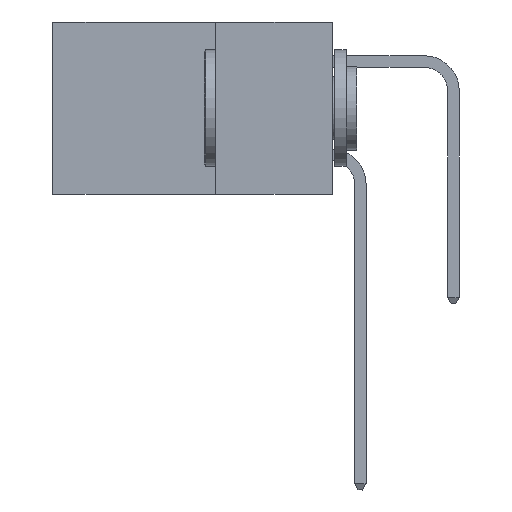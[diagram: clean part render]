
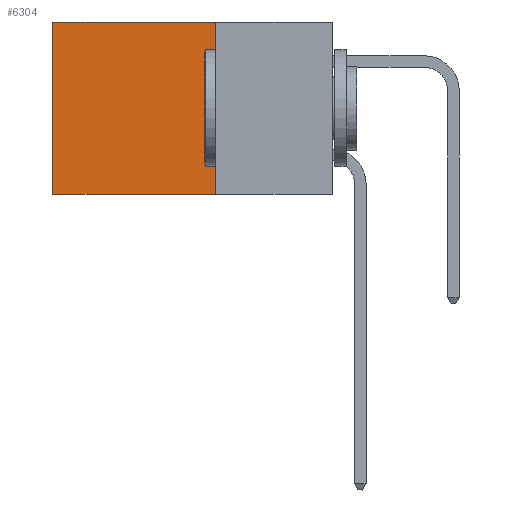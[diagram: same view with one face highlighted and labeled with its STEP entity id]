
A CAD part, left-side view. The second image highlights one B-rep face of the part: STEP entity #6304.
In plain terms, the highlighted planar face has unit normal (-1, 0, 0).
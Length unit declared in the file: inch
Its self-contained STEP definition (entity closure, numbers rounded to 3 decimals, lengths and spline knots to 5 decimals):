
#1602 = VERTEX_POINT ( 'NONE', #7469 ) ;
#1664 = LINE ( 'NONE', #8530, #12960 ) ;
#2072 = DIRECTION ( 'NONE',  ( 0., 1., 0. ) ) ;
#2282 = CARTESIAN_POINT ( 'NONE',  ( 0.298, 0.6, -0.37 ) ) ;
#2314 = VECTOR ( 'NONE', #13145, 39.37008 ) ;
#2537 = EDGE_CURVE ( 'NONE', #3053, #11686, #13222, .T. ) ;
#2742 = CARTESIAN_POINT ( 'NONE',  ( 0.298, 0.25, -0.37 ) ) ;
#2805 = CARTESIAN_POINT ( 'NONE',  ( 0.298, 0.25, 0. ) ) ;
#2840 = ORIENTED_EDGE ( 'NONE', *, *, #2537, .T. ) ;
#2880 = ORIENTED_EDGE ( 'NONE', *, *, #4846, .F. ) ;
#2893 = ORIENTED_EDGE ( 'NONE', *, *, #6145, .F. ) ;
#3053 = VERTEX_POINT ( 'NONE', #4993 ) ;
#3599 = ORIENTED_EDGE ( 'NONE', *, *, #12048, .T. ) ;
#3762 = DIRECTION ( 'NONE',  ( 0., 0., -1. ) ) ;
#4803 = EDGE_LOOP ( 'NONE', ( #2840, #2880, #2893, #3599 ) ) ;
#4846 = EDGE_CURVE ( 'NONE', #5453, #11686, #12691, .T. ) ;
#4993 = CARTESIAN_POINT ( 'NONE',  ( 0.298, 0.6, 0. ) ) ;
#5378 = CARTESIAN_POINT ( 'NONE',  ( 0.298, 0.25, 0. ) ) ;
#5381 = PLANE ( 'NONE',  #10415 ) ;
#5453 = VERTEX_POINT ( 'NONE', #10151 ) ;
#5815 = DIRECTION ( 'NONE',  ( 0., 0., -1. ) ) ;
#5863 = DIRECTION ( 'NONE',  ( 1., 0., 0. ) ) ;
#6082 = DIRECTION ( 'NONE',  ( 0., 1., 0. ) ) ;
#6145 = EDGE_CURVE ( 'NONE', #1602, #5453, #1664, .T. ) ;
#6304 = ADVANCED_FACE ( 'NONE', ( #13398 ), #5381, .F. ) ;
#7127 = VECTOR ( 'NONE', #2072, 39.37008 ) ;
#7469 = CARTESIAN_POINT ( 'NONE',  ( 0.298, 0.25, 0. ) ) ;
#8530 = CARTESIAN_POINT ( 'NONE',  ( 0.298, 0.25, 0. ) ) ;
#8979 = VECTOR ( 'NONE', #6082, 39.37008 ) ;
#10151 = CARTESIAN_POINT ( 'NONE',  ( 0.298, 0.25, -0.37 ) ) ;
#10415 = AXIS2_PLACEMENT_3D ( 'NONE', #5378, #5863, #5815 ) ;
#11686 = VERTEX_POINT ( 'NONE', #2282 ) ;
#11730 = LINE ( 'NONE', #2805, #8979 ) ;
#12048 = EDGE_CURVE ( 'NONE', #1602, #3053, #11730, .T. ) ;
#12691 = LINE ( 'NONE', #2742, #7127 ) ;
#12960 = VECTOR ( 'NONE', #3762, 39.37008 ) ;
#13145 = DIRECTION ( 'NONE',  ( 0., 0., -1. ) ) ;
#13171 = CARTESIAN_POINT ( 'NONE',  ( 0.298, 0.6, 0. ) ) ;
#13222 = LINE ( 'NONE', #13171, #2314 ) ;
#13398 = FACE_OUTER_BOUND ( 'NONE', #4803, .T. ) ;
